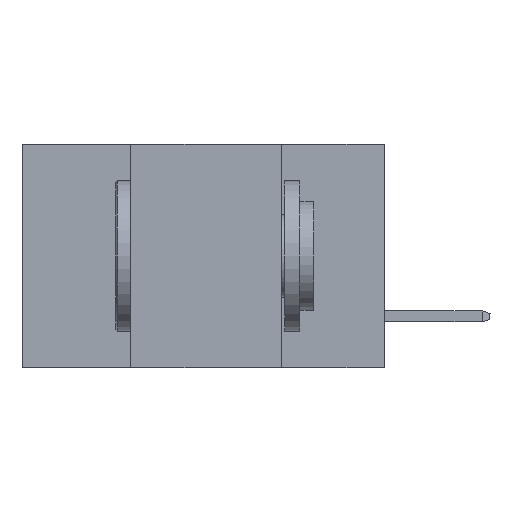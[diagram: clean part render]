
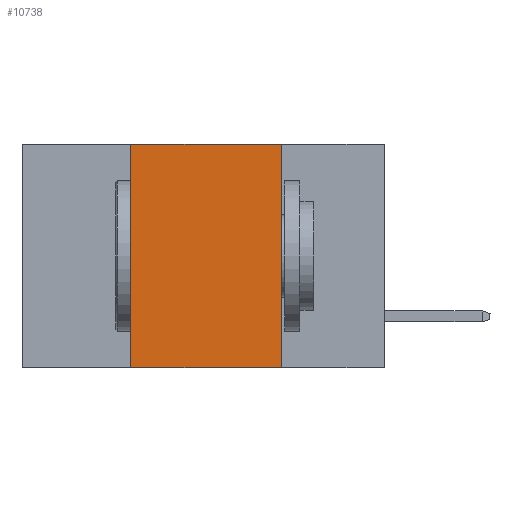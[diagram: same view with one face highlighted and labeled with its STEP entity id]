
A CAD part, left-side view. The second image highlights one B-rep face of the part: STEP entity #10738.
In plain terms, the highlighted planar face has unit normal (-1, 0, 0).
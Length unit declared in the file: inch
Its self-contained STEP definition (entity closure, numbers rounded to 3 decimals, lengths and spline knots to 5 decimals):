
#657 = CARTESIAN_POINT ( 'NONE',  ( 0., 0.42, -0.37 ) ) ;
#800 = CARTESIAN_POINT ( 'NONE',  ( 0., 0.6, 0. ) ) ;
#1020 = LINE ( 'NONE', #8732, #11617 ) ;
#1127 = CARTESIAN_POINT ( 'NONE',  ( 0., 0.42, 0. ) ) ;
#1480 = EDGE_CURVE ( 'NONE', #10635, #3773, #1020, .T. ) ;
#1916 = DIRECTION ( 'NONE',  ( 0., 0., -1. ) ) ;
#2678 = PLANE ( 'NONE',  #7096 ) ;
#2747 = FACE_OUTER_BOUND ( 'NONE', #5719, .T. ) ;
#3053 = LINE ( 'NONE', #800, #4754 ) ;
#3216 = CARTESIAN_POINT ( 'NONE',  ( 0., 0.17, 0. ) ) ;
#3271 = VERTEX_POINT ( 'NONE', #3216 ) ;
#3773 = VERTEX_POINT ( 'NONE', #11997 ) ;
#4754 = VECTOR ( 'NONE', #5704, 39.37008 ) ;
#4796 = LINE ( 'NONE', #7026, #5642 ) ;
#5503 = DIRECTION ( 'NONE',  ( 1., 0., 0. ) ) ;
#5642 = VECTOR ( 'NONE', #1916, 39.37008 ) ;
#5704 = DIRECTION ( 'NONE',  ( 0., -1., 0. ) ) ;
#5719 = EDGE_LOOP ( 'NONE', ( #6538, #9547, #7712, #7432 ) ) ;
#5867 = DIRECTION ( 'NONE',  ( 0., -1., 0. ) ) ;
#6105 = EDGE_CURVE ( 'NONE', #10635, #8677, #11949, .T. ) ;
#6435 = VECTOR ( 'NONE', #9283, 39.37008 ) ;
#6538 = ORIENTED_EDGE ( 'NONE', *, *, #10840, .F. ) ;
#7026 = CARTESIAN_POINT ( 'NONE',  ( 0., 0.17, -0.37 ) ) ;
#7096 = AXIS2_PLACEMENT_3D ( 'NONE', #8434, #5503, #9389 ) ;
#7432 = ORIENTED_EDGE ( 'NONE', *, *, #1480, .T. ) ;
#7712 = ORIENTED_EDGE ( 'NONE', *, *, #6105, .F. ) ;
#8139 = CARTESIAN_POINT ( 'NONE',  ( 0., 0.42, -0.37 ) ) ;
#8434 = CARTESIAN_POINT ( 'NONE',  ( 0., 0.6, 0. ) ) ;
#8677 = VERTEX_POINT ( 'NONE', #1127 ) ;
#8732 = CARTESIAN_POINT ( 'NONE',  ( 0., 0.6, -0.37 ) ) ;
#9283 = DIRECTION ( 'NONE',  ( 0., 0., 1. ) ) ;
#9389 = DIRECTION ( 'NONE',  ( 0., 0., -1. ) ) ;
#9547 = ORIENTED_EDGE ( 'NONE', *, *, #12064, .F. ) ;
#10635 = VERTEX_POINT ( 'NONE', #657 ) ;
#10738 = ADVANCED_FACE ( 'NONE', ( #2747 ), #2678, .F. ) ;
#10840 = EDGE_CURVE ( 'NONE', #3271, #3773, #4796, .T. ) ;
#11617 = VECTOR ( 'NONE', #5867, 39.37008 ) ;
#11949 = LINE ( 'NONE', #8139, #6435 ) ;
#11997 = CARTESIAN_POINT ( 'NONE',  ( 0., 0.17, -0.37 ) ) ;
#12064 = EDGE_CURVE ( 'NONE', #8677, #3271, #3053, .T. ) ;
